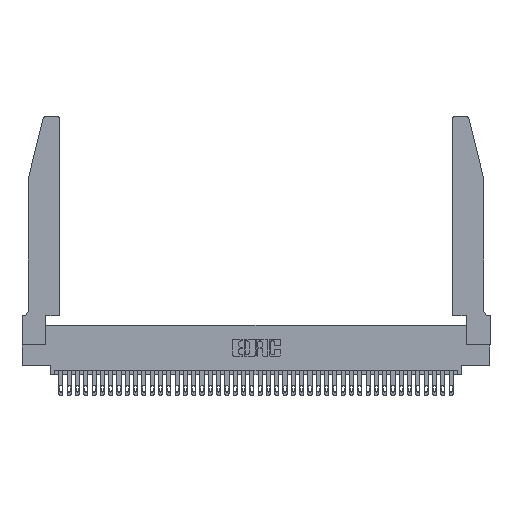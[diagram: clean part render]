
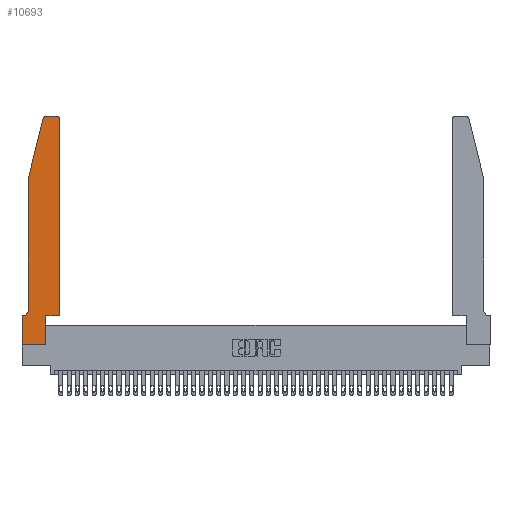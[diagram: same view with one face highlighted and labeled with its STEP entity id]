
A CAD part, top view. The second image highlights one B-rep face of the part: STEP entity #10693.
In plain terms, the highlighted planar face has unit normal (0, 0, 1).
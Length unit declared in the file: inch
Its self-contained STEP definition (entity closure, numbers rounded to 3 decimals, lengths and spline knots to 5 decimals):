
#93 = VERTEX_POINT ( 'NONE', #40876 ) ;
#474 = ORIENTED_EDGE ( 'NONE', *, *, #40297, .T. ) ;
#500 = VERTEX_POINT ( 'NONE', #11418 ) ;
#798 = CARTESIAN_POINT ( 'NONE',  ( 0.0755, 2., 0.37 ) ) ;
#833 = EDGE_CURVE ( 'NONE', #19871, #5835, #32170, .T. ) ;
#1352 = VERTEX_POINT ( 'NONE', #9239 ) ;
#1977 = EDGE_CURVE ( 'NONE', #31430, #5848, #17330, .T. ) ;
#2043 = EDGE_CURVE ( 'NONE', #1352, #500, #29393, .T. ) ;
#2260 = CARTESIAN_POINT ( 'NONE',  ( 0.2605, 2.75, 0.37 ) ) ;
#2387 = DIRECTION ( 'NONE',  ( -1., 0., 0. ) ) ;
#2413 = EDGE_CURVE ( 'NONE', #5835, #31430, #25350, .T. ) ;
#3035 = ORIENTED_EDGE ( 'NONE', *, *, #21820, .T. ) ;
#3581 = LINE ( 'NONE', #2260, #32814 ) ;
#3900 = CIRCLE ( 'NONE', #6003, 0.03 ) ;
#4090 = LINE ( 'NONE', #14041, #12187 ) ;
#4772 = ORIENTED_EDGE ( 'NONE', *, *, #8480, .T. ) ;
#4908 = CARTESIAN_POINT ( 'NONE',  ( 0.0755, 2., 0.37 ) ) ;
#5835 = VERTEX_POINT ( 'NONE', #33163 ) ;
#5848 = VERTEX_POINT ( 'NONE', #20949 ) ;
#6003 = AXIS2_PLACEMENT_3D ( 'NONE', #13029, #16264, #19498 ) ;
#6302 = ORIENTED_EDGE ( 'NONE', *, *, #1977, .T. ) ;
#6370 = EDGE_CURVE ( 'NONE', #5848, #93, #7584, .T. ) ;
#6952 = CARTESIAN_POINT ( 'NONE',  ( 0.4505, 0.35, 0.37 ) ) ;
#7584 = LINE ( 'NONE', #33115, #16152 ) ;
#7619 = CIRCLE ( 'NONE', #10220, 0.03 ) ;
#8444 = DIRECTION ( 'NONE',  ( -0.239, -0.971, 0. ) ) ;
#8480 = EDGE_CURVE ( 'NONE', #37508, #34516, #23368, .T. ) ;
#8646 = ORIENTED_EDGE ( 'NONE', *, *, #31533, .T. ) ;
#9239 = CARTESIAN_POINT ( 'NONE',  ( 0.2865, 0.35, 0.37 ) ) ;
#9846 = CARTESIAN_POINT ( 'NONE',  ( 0.0055, 0.42, 0.37 ) ) ;
#9873 = DIRECTION ( 'NONE',  ( 0., 1., 0. ) ) ;
#10220 = AXIS2_PLACEMENT_3D ( 'NONE', #14126, #36655, #17381 ) ;
#10693 = ADVANCED_FACE ( 'NONE', ( #12192 ), #25024, .T. ) ;
#10904 = CARTESIAN_POINT ( 'NONE',  ( 0.284, 2.75, 0.37 ) ) ;
#11418 = CARTESIAN_POINT ( 'NONE',  ( 0.4505, 0.35, 0.37 ) ) ;
#11795 = VECTOR ( 'NONE', #32448, 39.37008 ) ;
#12187 = VECTOR ( 'NONE', #30368, 39.37008 ) ;
#12192 = FACE_OUTER_BOUND ( 'NONE', #27706, .T. ) ;
#12306 = VECTOR ( 'NONE', #8444, 39.37008 ) ;
#12373 = DIRECTION ( 'NONE',  ( 0., 0., 1. ) ) ;
#12555 = CARTESIAN_POINT ( 'NONE',  ( 0., 0.35, 0.37 ) ) ;
#13029 = CARTESIAN_POINT ( 'NONE',  ( 0.284, 2.72, 0.37 ) ) ;
#14041 = CARTESIAN_POINT ( 'NONE',  ( 0.4505, 0.35, 0.37 ) ) ;
#14126 = CARTESIAN_POINT ( 'NONE',  ( 0.4205, 2.72, 0.37 ) ) ;
#14151 = ORIENTED_EDGE ( 'NONE', *, *, #2043, .T. ) ;
#15574 = CARTESIAN_POINT ( 'NONE',  ( 0., 0., 0.37 ) ) ;
#16152 = VECTOR ( 'NONE', #20469, 39.37008 ) ;
#16264 = DIRECTION ( 'NONE',  ( 0., 0., 1. ) ) ;
#17092 = EDGE_CURVE ( 'NONE', #34516, #19871, #29938, .T. ) ;
#17330 = LINE ( 'NONE', #15574, #31421 ) ;
#17381 = DIRECTION ( 'NONE',  ( 1., 0., 0. ) ) ;
#17886 = ORIENTED_EDGE ( 'NONE', *, *, #6370, .T. ) ;
#19498 = DIRECTION ( 'NONE',  ( 1., 0., 0. ) ) ;
#19871 = VERTEX_POINT ( 'NONE', #34406 ) ;
#19924 = VECTOR ( 'NONE', #9873, 39.37008 ) ;
#20469 = DIRECTION ( 'NONE',  ( 1., 0., 0. ) ) ;
#20949 = CARTESIAN_POINT ( 'NONE',  ( 0., 0., 0.37 ) ) ;
#21120 = AXIS2_PLACEMENT_3D ( 'NONE', #38267, #12373, #31787 ) ;
#21820 = EDGE_CURVE ( 'NONE', #23837, #37508, #3900, .T. ) ;
#23368 = LINE ( 'NONE', #4908, #12306 ) ;
#23397 = VECTOR ( 'NONE', #26699, 39.37008 ) ;
#23837 = VERTEX_POINT ( 'NONE', #10904 ) ;
#24340 = VECTOR ( 'NONE', #34708, 39.37008 ) ;
#25024 = PLANE ( 'NONE',  #21120 ) ;
#25350 = LINE ( 'NONE', #31743, #24340 ) ;
#25513 = ORIENTED_EDGE ( 'NONE', *, *, #35600, .T. ) ;
#25967 = ORIENTED_EDGE ( 'NONE', *, *, #40965, .T. ) ;
#26223 = ORIENTED_EDGE ( 'NONE', *, *, #833, .T. ) ;
#26326 = CARTESIAN_POINT ( 'NONE',  ( 0.4505, 2.72, 0.37 ) ) ;
#26524 = LINE ( 'NONE', #29283, #19924 ) ;
#26567 = AXIS2_PLACEMENT_3D ( 'NONE', #9846, #39110, #26864 ) ;
#26667 = CARTESIAN_POINT ( 'NONE',  ( 0.25487, 2.72718, 0.37 ) ) ;
#26699 = DIRECTION ( 'NONE',  ( 0., -1., 0. ) ) ;
#26864 = DIRECTION ( 'NONE',  ( -1., 0., 0. ) ) ;
#27706 = EDGE_LOOP ( 'NONE', ( #25513, #3035, #4772, #31402, #26223, #35076, #6302, #17886, #8646, #14151, #474, #25967 ) ) ;
#28946 = CARTESIAN_POINT ( 'NONE',  ( 0.0755, 2., 0.37 ) ) ;
#29283 = CARTESIAN_POINT ( 'NONE',  ( 0.2865, 0.35, 0.37 ) ) ;
#29393 = LINE ( 'NONE', #6952, #11795 ) ;
#29938 = LINE ( 'NONE', #798, #23397 ) ;
#30368 = DIRECTION ( 'NONE',  ( 0., 1., 0. ) ) ;
#31402 = ORIENTED_EDGE ( 'NONE', *, *, #17092, .T. ) ;
#31421 = VECTOR ( 'NONE', #31911, 39.37008 ) ;
#31430 = VERTEX_POINT ( 'NONE', #12555 ) ;
#31533 = EDGE_CURVE ( 'NONE', #93, #1352, #26524, .T. ) ;
#31743 = CARTESIAN_POINT ( 'NONE',  ( 0.0755, 0.35, 0.37 ) ) ;
#31787 = DIRECTION ( 'NONE',  ( 1., 0., 0. ) ) ;
#31911 = DIRECTION ( 'NONE',  ( 0., -1., 0. ) ) ;
#32170 = CIRCLE ( 'NONE', #26567, 0.07 ) ;
#32448 = DIRECTION ( 'NONE',  ( 1., 0., 0. ) ) ;
#32649 = CARTESIAN_POINT ( 'NONE',  ( 0.4205, 2.75, 0.37 ) ) ;
#32814 = VECTOR ( 'NONE', #2387, 39.37008 ) ;
#33115 = CARTESIAN_POINT ( 'NONE',  ( 0., 0., 0.37 ) ) ;
#33163 = CARTESIAN_POINT ( 'NONE',  ( 0.0055, 0.35, 0.37 ) ) ;
#33491 = VERTEX_POINT ( 'NONE', #26326 ) ;
#34406 = CARTESIAN_POINT ( 'NONE',  ( 0.0755, 0.42, 0.37 ) ) ;
#34516 = VERTEX_POINT ( 'NONE', #28946 ) ;
#34708 = DIRECTION ( 'NONE',  ( -1., 0., 0. ) ) ;
#35076 = ORIENTED_EDGE ( 'NONE', *, *, #2413, .T. ) ;
#35600 = EDGE_CURVE ( 'NONE', #40296, #23837, #3581, .T. ) ;
#36655 = DIRECTION ( 'NONE',  ( 0., 0., 1. ) ) ;
#37508 = VERTEX_POINT ( 'NONE', #26667 ) ;
#38267 = CARTESIAN_POINT ( 'NONE',  ( 0., 0.35, 0.37 ) ) ;
#39110 = DIRECTION ( 'NONE',  ( 0., 0., -1. ) ) ;
#40296 = VERTEX_POINT ( 'NONE', #32649 ) ;
#40297 = EDGE_CURVE ( 'NONE', #500, #33491, #4090, .T. ) ;
#40876 = CARTESIAN_POINT ( 'NONE',  ( 0.2865, 0., 0.37 ) ) ;
#40965 = EDGE_CURVE ( 'NONE', #33491, #40296, #7619, .T. ) ;
